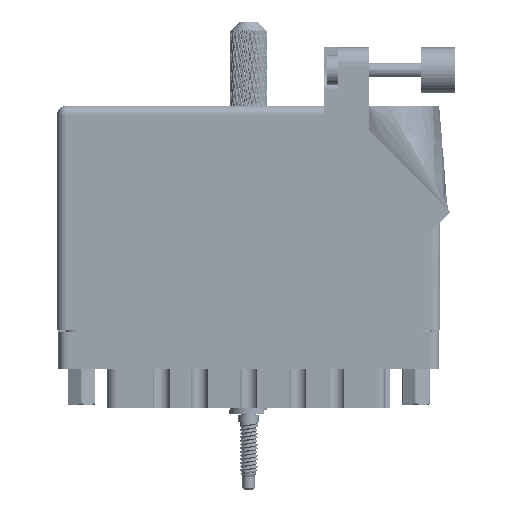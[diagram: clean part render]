
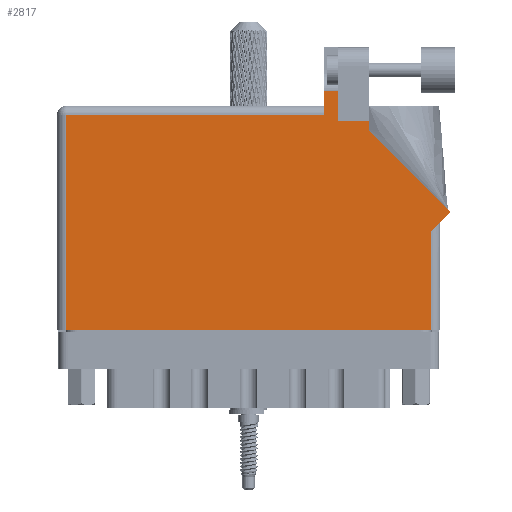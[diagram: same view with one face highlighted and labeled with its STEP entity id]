
A CAD part, front view. The second image highlights one B-rep face of the part: STEP entity #2817.
In plain terms, the highlighted face is planar.
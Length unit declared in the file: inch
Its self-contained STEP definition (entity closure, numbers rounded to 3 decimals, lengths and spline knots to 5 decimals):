
#2106 = LINE ( 'NONE', #75289, #113644 ) ;
#2817 = ADVANCED_FACE ( 'NONE', ( #4084 ), #38707, .F. ) ;
#4084 = FACE_OUTER_BOUND ( 'NONE', #75254, .T. ) ;
#5694 = CARTESIAN_POINT ( 'NONE',  ( 1.913, 1.43, 0. ) ) ;
#6332 = CARTESIAN_POINT ( 'NONE',  ( 1.913, 1.6315, 0. ) ) ;
#6910 = ORIENTED_EDGE ( 'NONE', *, *, #42896, .T. ) ;
#8119 = CARTESIAN_POINT ( 'NONE',  ( 0.062, 1.468, 0. ) ) ;
#8655 = CARTESIAN_POINT ( 'NONE',  ( 2.68271, 0.80771, 0. ) ) ;
#9871 = CARTESIAN_POINT ( 'NONE',  ( 2.55, 0.737, 0. ) ) ;
#14636 = VECTOR ( 'NONE', #64186, 39.37008 ) ;
#18779 = DIRECTION ( 'NONE',  ( 0., 0., -1. ) ) ;
#20833 = VECTOR ( 'NONE', #119886, 39.37008 ) ;
#21901 = EDGE_CURVE ( 'NONE', #123759, #51802, #40983, .T. ) ;
#23171 = VECTOR ( 'NONE', #112463, 39.37008 ) ;
#23922 = CARTESIAN_POINT ( 'NONE',  ( 1.819, 1.468, 0. ) ) ;
#27535 = CARTESIAN_POINT ( 'NONE',  ( 2.55, 0., 0. ) ) ;
#29005 = LINE ( 'NONE', #9871, #32065 ) ;
#30764 = LINE ( 'NONE', #52948, #40052 ) ;
#32065 = VECTOR ( 'NONE', #60407, 39.37008 ) ;
#33089 = ORIENTED_EDGE ( 'NONE', *, *, #107588, .T. ) ;
#33916 = VERTEX_POINT ( 'NONE', #8655 ) ;
#34892 = DIRECTION ( 'NONE',  ( -1., 0., 0. ) ) ;
#35613 = LINE ( 'NONE', #97883, #97551 ) ;
#37927 = LINE ( 'NONE', #90801, #20833 ) ;
#38707 = PLANE ( 'NONE',  #50505 ) ;
#39300 = CARTESIAN_POINT ( 'NONE',  ( 1.819, 1.6315, 0. ) ) ;
#40052 = VECTOR ( 'NONE', #94070, 39.37008 ) ;
#40983 = LINE ( 'NONE', #91490, #14636 ) ;
#41560 = CARTESIAN_POINT ( 'NONE',  ( 2.612, 0.737, 0. ) ) ;
#42896 = EDGE_CURVE ( 'NONE', #92763, #103550, #35613, .T. ) ;
#43751 = VERTEX_POINT ( 'NONE', #6332 ) ;
#45177 = ORIENTED_EDGE ( 'NONE', *, *, #89119, .T. ) ;
#47835 = EDGE_CURVE ( 'NONE', #108991, #92763, #37927, .T. ) ;
#47984 = EDGE_CURVE ( 'NONE', #119556, #123759, #84313, .T. ) ;
#48220 = CARTESIAN_POINT ( 'NONE',  ( 0., 1.53, 0. ) ) ;
#50505 = AXIS2_PLACEMENT_3D ( 'NONE', #48220, #18779, #107956 ) ;
#51802 = VERTEX_POINT ( 'NONE', #78053 ) ;
#52948 = CARTESIAN_POINT ( 'NONE',  ( 2.24377, 1.6315, 0. ) ) ;
#54923 = CARTESIAN_POINT ( 'NONE',  ( 2.126, 1.36442, 0. ) ) ;
#56448 = VECTOR ( 'NONE', #92576, 39.37008 ) ;
#58000 = CARTESIAN_POINT ( 'NONE',  ( 2.126, 1.43, 0. ) ) ;
#58356 = VERTEX_POINT ( 'NONE', #65936 ) ;
#58613 = EDGE_CURVE ( 'NONE', #103550, #43751, #97601, .T. ) ;
#60407 = DIRECTION ( 'NONE',  ( 0., 1., 0. ) ) ;
#63774 = ORIENTED_EDGE ( 'NONE', *, *, #47984, .T. ) ;
#64186 = DIRECTION ( 'NONE',  ( 0., -1., 0. ) ) ;
#64537 = VERTEX_POINT ( 'NONE', #39300 ) ;
#64993 = LINE ( 'NONE', #92544, #23171 ) ;
#65936 = CARTESIAN_POINT ( 'NONE',  ( 2.55, 0.675, 0. ) ) ;
#67305 = ORIENTED_EDGE ( 'NONE', *, *, #21901, .T. ) ;
#73065 = CARTESIAN_POINT ( 'NONE',  ( 1.819, 1.53, 0. ) ) ;
#73439 = CARTESIAN_POINT ( 'NONE',  ( 0., 1.468, 0. ) ) ;
#75254 = EDGE_LOOP ( 'NONE', ( #82363, #101854, #82005, #63774, #67305, #45177, #33089, #116446, #103660, #111588, #6910 ) ) ;
#75289 = CARTESIAN_POINT ( 'NONE',  ( 0., 0., 0. ) ) ;
#78053 = CARTESIAN_POINT ( 'NONE',  ( 0.062, 0., 0. ) ) ;
#79888 = EDGE_CURVE ( 'NONE', #43751, #64537, #30764, .T. ) ;
#82005 = ORIENTED_EDGE ( 'NONE', *, *, #83873, .T. ) ;
#82363 = ORIENTED_EDGE ( 'NONE', *, *, #58613, .T. ) ;
#82720 = LINE ( 'NONE', #73065, #56448 ) ;
#83873 = EDGE_CURVE ( 'NONE', #64537, #119556, #82720, .T. ) ;
#84313 = LINE ( 'NONE', #73439, #87401 ) ;
#85669 = DIRECTION ( 'NONE',  ( 1., 0., 0. ) ) ;
#87401 = VECTOR ( 'NONE', #103751, 39.37008 ) ;
#89119 = EDGE_CURVE ( 'NONE', #51802, #127894, #2106, .T. ) ;
#90801 = CARTESIAN_POINT ( 'NONE',  ( 2.126, 1.36442, 0. ) ) ;
#91490 = CARTESIAN_POINT ( 'NONE',  ( 0.062, 0., 0. ) ) ;
#92544 = CARTESIAN_POINT ( 'NONE',  ( 2.68271, 0.80771, 0. ) ) ;
#92576 = DIRECTION ( 'NONE',  ( 0., -1., 0. ) ) ;
#92763 = VERTEX_POINT ( 'NONE', #58000 ) ;
#93110 = LINE ( 'NONE', #41560, #110146 ) ;
#93963 = DIRECTION ( 'NONE',  ( 0., 1., 0. ) ) ;
#94070 = DIRECTION ( 'NONE',  ( -1., 0., 0. ) ) ;
#95121 = CARTESIAN_POINT ( 'NONE',  ( 1.913, 1.43, 0. ) ) ;
#97551 = VECTOR ( 'NONE', #34892, 39.37008 ) ;
#97601 = LINE ( 'NONE', #5694, #99214 ) ;
#97883 = CARTESIAN_POINT ( 'NONE',  ( 2.126, 1.43, 0. ) ) ;
#99214 = VECTOR ( 'NONE', #93963, 39.37008 ) ;
#101262 = DIRECTION ( 'NONE',  ( 0.707, 0.707, 0. ) ) ;
#101854 = ORIENTED_EDGE ( 'NONE', *, *, #79888, .T. ) ;
#102931 = EDGE_CURVE ( 'NONE', #58356, #33916, #93110, .T. ) ;
#103550 = VERTEX_POINT ( 'NONE', #95121 ) ;
#103660 = ORIENTED_EDGE ( 'NONE', *, *, #116448, .T. ) ;
#103751 = DIRECTION ( 'NONE',  ( -1., 0., 0. ) ) ;
#107588 = EDGE_CURVE ( 'NONE', #127894, #58356, #29005, .T. ) ;
#107956 = DIRECTION ( 'NONE',  ( -1., 0., 0. ) ) ;
#108991 = VERTEX_POINT ( 'NONE', #54923 ) ;
#110146 = VECTOR ( 'NONE', #101262, 39.37008 ) ;
#111588 = ORIENTED_EDGE ( 'NONE', *, *, #47835, .T. ) ;
#112463 = DIRECTION ( 'NONE',  ( -0.707, 0.707, 0. ) ) ;
#113644 = VECTOR ( 'NONE', #85669, 39.37008 ) ;
#116446 = ORIENTED_EDGE ( 'NONE', *, *, #102931, .T. ) ;
#116448 = EDGE_CURVE ( 'NONE', #33916, #108991, #64993, .T. ) ;
#119556 = VERTEX_POINT ( 'NONE', #23922 ) ;
#119886 = DIRECTION ( 'NONE',  ( 0., 1., 0. ) ) ;
#123759 = VERTEX_POINT ( 'NONE', #8119 ) ;
#127894 = VERTEX_POINT ( 'NONE', #27535 ) ;
